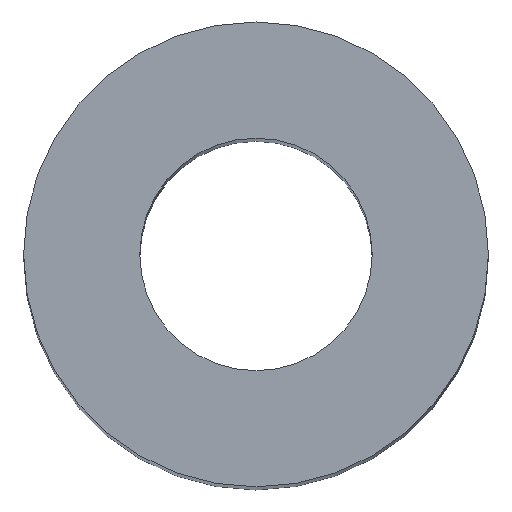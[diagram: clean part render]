
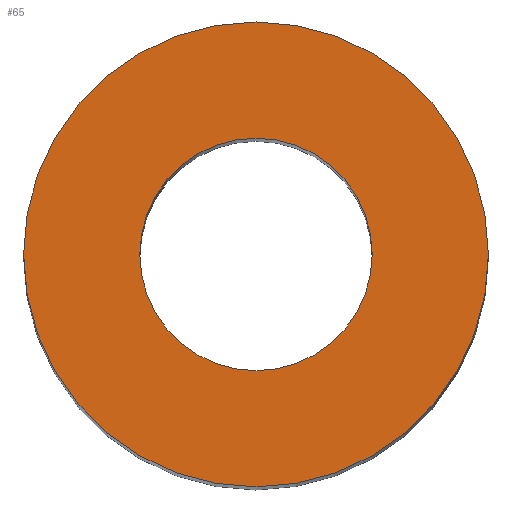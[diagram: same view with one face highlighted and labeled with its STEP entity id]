
A CAD part, top view. The second image highlights one B-rep face of the part: STEP entity #65.
In plain terms, the highlighted planar face has unit normal (0, 0, 1).
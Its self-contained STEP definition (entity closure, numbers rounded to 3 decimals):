
#3 = VERTEX_POINT ( 'NONE', #17 ) ;
#4 = DIRECTION ( 'NONE',  ( 1., 0., 0. ) ) ;
#5 = AXIS2_PLACEMENT_3D ( 'NONE', #54, #160, #60 ) ;
#14 = ORIENTED_EDGE ( 'NONE', *, *, #78, .T. ) ;
#17 = CARTESIAN_POINT ( 'NONE',  ( 3.5, 0., 27. ) ) ;
#22 = DIRECTION ( 'NONE',  ( 0., 0., 1. ) ) ;
#23 = AXIS2_PLACEMENT_3D ( 'NONE', #113, #22, #131 ) ;
#25 = EDGE_LOOP ( 'NONE', ( #129, #153 ) ) ;
#33 = CARTESIAN_POINT ( 'NONE',  ( 0., 0., 27. ) ) ;
#35 = AXIS2_PLACEMENT_3D ( 'NONE', #202, #90, #4 ) ;
#45 = FACE_OUTER_BOUND ( 'NONE', #88, .T. ) ;
#51 = DIRECTION ( 'NONE',  ( 1., 0., 0. ) ) ;
#54 = CARTESIAN_POINT ( 'NONE',  ( 0., 0., 27. ) ) ;
#56 = AXIS2_PLACEMENT_3D ( 'NONE', #67, #116, #205 ) ;
#60 = DIRECTION ( 'NONE',  ( 1., 0., 0. ) ) ;
#65 = ADVANCED_FACE ( 'NONE', ( #45, #84 ), #162, .T. ) ;
#67 = CARTESIAN_POINT ( 'NONE',  ( 0., 0., 27. ) ) ;
#68 = AXIS2_PLACEMENT_3D ( 'NONE', #33, #134, #51 ) ;
#74 = CARTESIAN_POINT ( 'NONE',  ( -3.5, 0., 27. ) ) ;
#78 = EDGE_CURVE ( 'NONE', #3, #80, #209, .T. ) ;
#79 = ORIENTED_EDGE ( 'NONE', *, *, #102, .T. ) ;
#80 = VERTEX_POINT ( 'NONE', #74 ) ;
#84 = FACE_BOUND ( 'NONE', #25, .T. ) ;
#86 = CARTESIAN_POINT ( 'NONE',  ( -1.75, 0., 27. ) ) ;
#88 = EDGE_LOOP ( 'NONE', ( #79, #14 ) ) ;
#90 = DIRECTION ( 'NONE',  ( 0., 0., 1. ) ) ;
#102 = EDGE_CURVE ( 'NONE', #80, #3, #181, .T. ) ;
#105 = EDGE_CURVE ( 'NONE', #135, #192, #184, .T. ) ;
#113 = CARTESIAN_POINT ( 'NONE',  ( 0., 0., 27. ) ) ;
#116 = DIRECTION ( 'NONE',  ( 0., 0., 1. ) ) ;
#129 = ORIENTED_EDGE ( 'NONE', *, *, #155, .F. ) ;
#131 = DIRECTION ( 'NONE',  ( 1., 0., 0. ) ) ;
#134 = DIRECTION ( 'NONE',  ( 0., 0., 1. ) ) ;
#135 = VERTEX_POINT ( 'NONE', #142 ) ;
#142 = CARTESIAN_POINT ( 'NONE',  ( 1.75, 0., 27. ) ) ;
#153 = ORIENTED_EDGE ( 'NONE', *, *, #105, .F. ) ;
#155 = EDGE_CURVE ( 'NONE', #192, #135, #157, .T. ) ;
#157 = CIRCLE ( 'NONE', #5, 1.75 ) ;
#160 = DIRECTION ( 'NONE',  ( 0., 0., 1. ) ) ;
#162 = PLANE ( 'NONE',  #56 ) ;
#181 = CIRCLE ( 'NONE', #23, 3.5 ) ;
#184 = CIRCLE ( 'NONE', #35, 1.75 ) ;
#192 = VERTEX_POINT ( 'NONE', #86 ) ;
#202 = CARTESIAN_POINT ( 'NONE',  ( 0., 0., 27. ) ) ;
#205 = DIRECTION ( 'NONE',  ( 1., 0., 0. ) ) ;
#209 = CIRCLE ( 'NONE', #68, 3.5 ) ;
